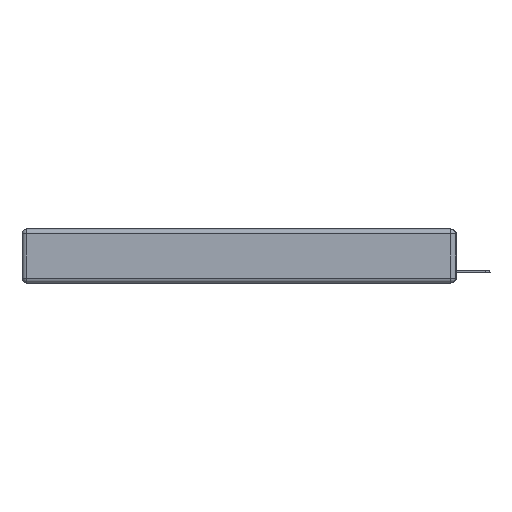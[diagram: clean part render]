
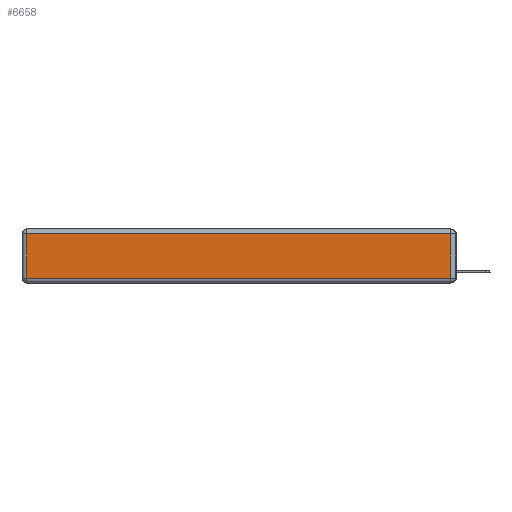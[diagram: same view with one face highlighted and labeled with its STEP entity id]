
A CAD part, left-side view. The second image highlights one B-rep face of the part: STEP entity #6658.
In plain terms, the highlighted planar face has unit normal (-1, 0, 0).
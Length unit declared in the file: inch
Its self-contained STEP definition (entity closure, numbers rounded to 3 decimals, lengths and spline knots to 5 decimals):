
#213 = VERTEX_POINT ( 'NONE', #20837 ) ;
#679 = VECTOR ( 'NONE', #4155, 39.37008 ) ;
#1019 = VERTEX_POINT ( 'NONE', #12087 ) ;
#2302 = FACE_OUTER_BOUND ( 'NONE', #7828, .T. ) ;
#4155 = DIRECTION ( 'NONE',  ( 0., 1., 0. ) ) ;
#4205 = DIRECTION ( 'NONE',  ( 0., 0., 1. ) ) ;
#4347 = ORIENTED_EDGE ( 'NONE', *, *, #20497, .T. ) ;
#4957 = LINE ( 'NONE', #10386, #20385 ) ;
#6086 = VECTOR ( 'NONE', #4205, 39.37008 ) ;
#6658 = ADVANCED_FACE ( 'NONE', ( #2302 ), #8848, .T. ) ;
#7165 = VECTOR ( 'NONE', #16651, 39.37008 ) ;
#7828 = EDGE_LOOP ( 'NONE', ( #15048, #4347, #14948, #7972 ) ) ;
#7905 = LINE ( 'NONE', #19806, #679 ) ;
#7972 = ORIENTED_EDGE ( 'NONE', *, *, #8088, .T. ) ;
#8088 = EDGE_CURVE ( 'NONE', #1019, #13709, #4957, .T. ) ;
#8801 = AXIS2_PLACEMENT_3D ( 'NONE', #15627, #14072, #17078 ) ;
#8848 = PLANE ( 'NONE',  #8801 ) ;
#9293 = EDGE_CURVE ( 'NONE', #13709, #11876, #13305, .T. ) ;
#10386 = CARTESIAN_POINT ( 'NONE',  ( 0., 2.72, -0.343 ) ) ;
#11075 = LINE ( 'NONE', #16091, #6086 ) ;
#11876 = VERTEX_POINT ( 'NONE', #14918 ) ;
#12087 = CARTESIAN_POINT ( 'NONE',  ( 0., 2.72, -0.03 ) ) ;
#13305 = LINE ( 'NONE', #14874, #7165 ) ;
#13709 = VERTEX_POINT ( 'NONE', #18780 ) ;
#13716 = DIRECTION ( 'NONE',  ( 0., 0., -1. ) ) ;
#14072 = DIRECTION ( 'NONE',  ( -1., 0., 0. ) ) ;
#14874 = CARTESIAN_POINT ( 'NONE',  ( 0., 0., -0.313 ) ) ;
#14918 = CARTESIAN_POINT ( 'NONE',  ( 0., 0.03, -0.313 ) ) ;
#14948 = ORIENTED_EDGE ( 'NONE', *, *, #18529, .T. ) ;
#15048 = ORIENTED_EDGE ( 'NONE', *, *, #9293, .T. ) ;
#15627 = CARTESIAN_POINT ( 'NONE',  ( 0., 0., -0.343 ) ) ;
#16091 = CARTESIAN_POINT ( 'NONE',  ( 0., 0.03, -0.343 ) ) ;
#16651 = DIRECTION ( 'NONE',  ( 0., -1., 0. ) ) ;
#17078 = DIRECTION ( 'NONE',  ( 0., 0., 1. ) ) ;
#18529 = EDGE_CURVE ( 'NONE', #213, #1019, #7905, .T. ) ;
#18780 = CARTESIAN_POINT ( 'NONE',  ( 0., 2.72, -0.313 ) ) ;
#19806 = CARTESIAN_POINT ( 'NONE',  ( 0., 2.75, -0.03 ) ) ;
#20385 = VECTOR ( 'NONE', #13716, 39.37008 ) ;
#20497 = EDGE_CURVE ( 'NONE', #11876, #213, #11075, .T. ) ;
#20837 = CARTESIAN_POINT ( 'NONE',  ( 0., 0.03, -0.03 ) ) ;
